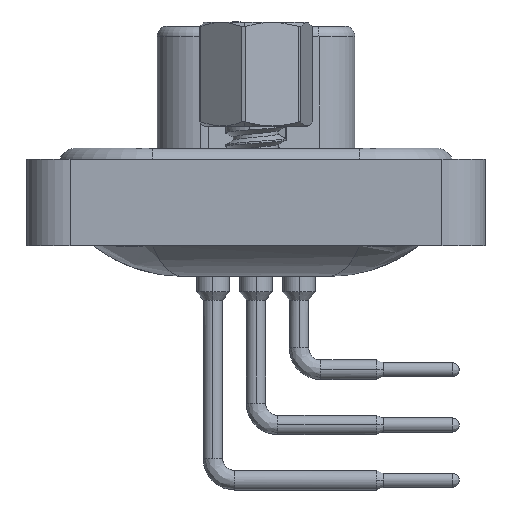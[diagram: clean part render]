
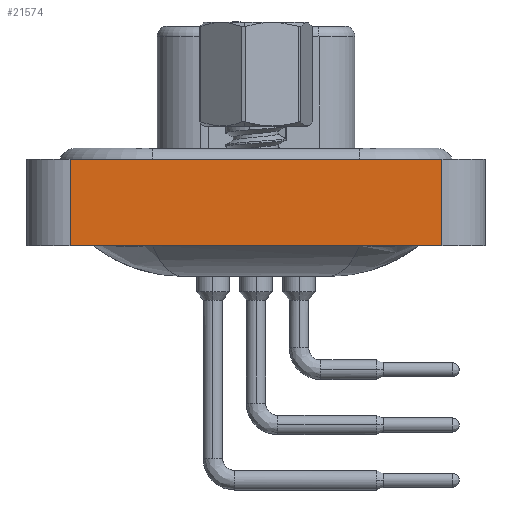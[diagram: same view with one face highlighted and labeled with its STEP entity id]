
A CAD part, left-side view. The second image highlights one B-rep face of the part: STEP entity #21574.
In plain terms, the highlighted planar face has unit normal (-1, 0, 0).
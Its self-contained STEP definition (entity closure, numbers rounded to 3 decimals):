
#7 = EDGE_CURVE ( 'NONE', #26528, #17442, #27005, .T. ) ;
#1405 = VERTEX_POINT ( 'NONE', #25211 ) ;
#3893 = EDGE_CURVE ( 'NONE', #26528, #1405, #26728, .T. ) ;
#4302 = CARTESIAN_POINT ( 'NONE',  ( -7.26, -8.55, 0.4 ) ) ;
#5197 = LINE ( 'NONE', #17218, #15972 ) ;
#5328 = ORIENTED_EDGE ( 'NONE', *, *, #9874, .F. ) ;
#5909 = EDGE_CURVE ( 'NONE', #17442, #14735, #5197, .T. ) ;
#6494 = PLANE ( 'NONE',  #29947 ) ;
#6521 = VECTOR ( 'NONE', #25888, 1000. ) ;
#6760 = LINE ( 'NONE', #4302, #6521 ) ;
#6945 = DIRECTION ( 'NONE',  ( 0., 0., 1. ) ) ;
#8907 = CARTESIAN_POINT ( 'NONE',  ( -7.26, -8.55, 0.4 ) ) ;
#9099 = ORIENTED_EDGE ( 'NONE', *, *, #3893, .F. ) ;
#9874 = EDGE_CURVE ( 'NONE', #1405, #14735, #6760, .T. ) ;
#11707 = VECTOR ( 'NONE', #17407, 1000. ) ;
#12145 = DIRECTION ( 'NONE',  ( 0., 0., 1. ) ) ;
#12646 = CARTESIAN_POINT ( 'NONE',  ( -7.26, -8.55, -3.6 ) ) ;
#14051 = CARTESIAN_POINT ( 'NONE',  ( -7.26, 8.55, -3.6 ) ) ;
#14183 = FACE_OUTER_BOUND ( 'NONE', #18467, .T. ) ;
#14735 = VERTEX_POINT ( 'NONE', #8907 ) ;
#15069 = VECTOR ( 'NONE', #23378, 1000. ) ;
#15972 = VECTOR ( 'NONE', #12145, 1000. ) ;
#17218 = CARTESIAN_POINT ( 'NONE',  ( -7.26, -8.55, -3.6 ) ) ;
#17407 = DIRECTION ( 'NONE',  ( 0., -1., 0. ) ) ;
#17442 = VERTEX_POINT ( 'NONE', #26218 ) ;
#18467 = EDGE_LOOP ( 'NONE', ( #24315, #5328, #9099, #19078 ) ) ;
#18518 = DIRECTION ( 'NONE',  ( -1., 0., 0. ) ) ;
#19078 = ORIENTED_EDGE ( 'NONE', *, *, #7, .T. ) ;
#21574 = ADVANCED_FACE ( 'NONE', ( #14183 ), #6494, .T. ) ;
#23378 = DIRECTION ( 'NONE',  ( 0., 0., 1. ) ) ;
#24315 = ORIENTED_EDGE ( 'NONE', *, *, #5909, .T. ) ;
#25211 = CARTESIAN_POINT ( 'NONE',  ( -7.26, 8.55, 0.4 ) ) ;
#25888 = DIRECTION ( 'NONE',  ( 0., -1., 0. ) ) ;
#26218 = CARTESIAN_POINT ( 'NONE',  ( -7.26, -8.55, -3.6 ) ) ;
#26411 = CARTESIAN_POINT ( 'NONE',  ( -7.26, 8.55, -3.6 ) ) ;
#26528 = VERTEX_POINT ( 'NONE', #14051 ) ;
#26728 = LINE ( 'NONE', #26411, #15069 ) ;
#27005 = LINE ( 'NONE', #12646, #11707 ) ;
#29947 = AXIS2_PLACEMENT_3D ( 'NONE', #30135, #18518, #6945 ) ;
#30135 = CARTESIAN_POINT ( 'NONE',  ( -7.26, -8.55, -3.6 ) ) ;
